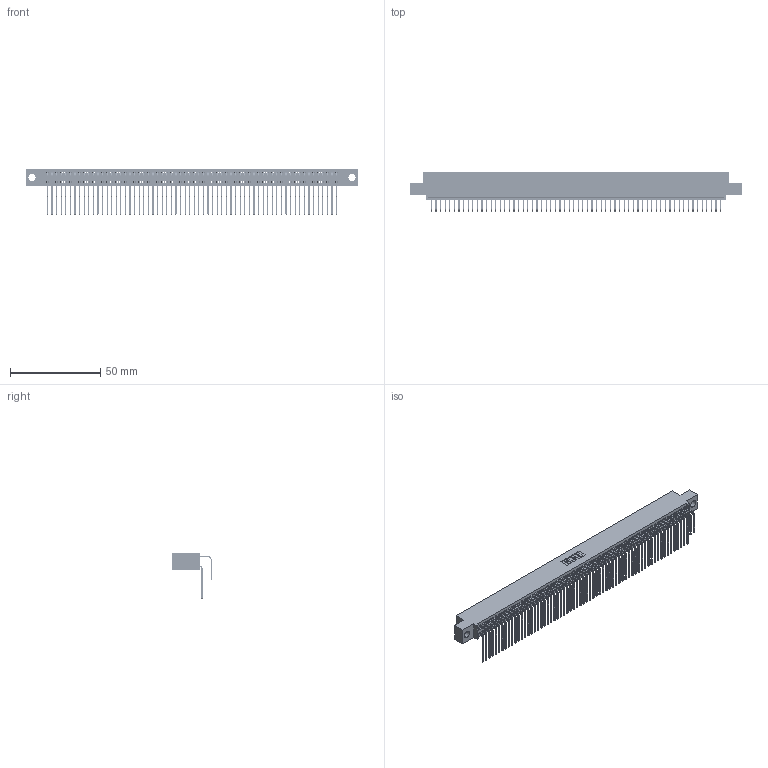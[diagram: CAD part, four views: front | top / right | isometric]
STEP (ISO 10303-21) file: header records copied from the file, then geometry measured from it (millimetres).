
FILE_DESCRIPTION (( 'STEP AP203' ), '1' );
FILE_NAME ('395-128-558-504.STEP', '2021-06-17T23:53:56', ( '' ), ( '' ), 'SwSTEP 2.0', 'SolidWorks 2020', '' );
FILE_SCHEMA (( 'CONFIG_CONTROL_DESIGN' ));
Length unit declared in the file: inch
Products named in the file (4): 345-292-001_558 559 Tail - 1; 395-128-558-504; 345 Part_0.110 Offset - 0.156 Dia-TI; 345-292-001_558 Tail - 2
Assembly tree (129 placements, depth 2):
  395-128-558-504
    345 Part_0.110 Offset - 0.156 Dia-TI
    345-292-001_558 559 Tail - 1  x64
    345-292-001_558 Tail - 2  x64
Bounding box: 183.77 x 21.83 x 25.53 mm (x, y, z)
Volume: 18614.8 mm3; surface area: 31358.5 mm2
Topology: 129 solids, 129 shells, 6800 faces, 20229 edges, 13314 vertices
Faces by surface type: plane 4578, cylinder 2222
Entity records: 49457 total; most frequent: CARTESIAN_POINT 8321, ORIENTED_EDGE 8202, DIRECTION 7281, EDGE_CURVE 4101, LINE 3673, VECTOR 3673, VERTEX_POINT 2730, AXIS2_PLACEMENT_3D 1804
